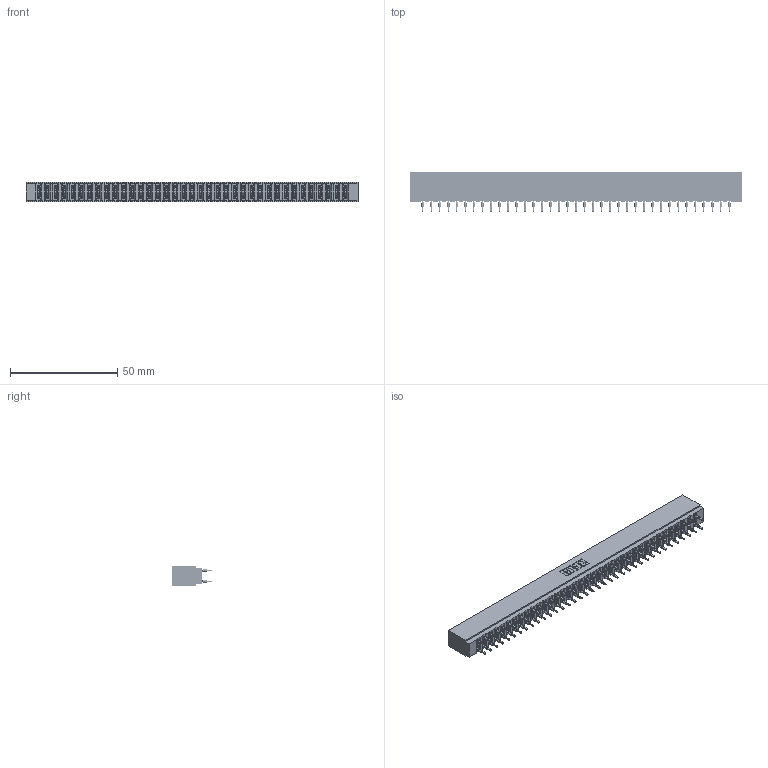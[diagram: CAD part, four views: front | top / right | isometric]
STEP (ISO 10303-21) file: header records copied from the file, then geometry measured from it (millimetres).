
FILE_DESCRIPTION (( 'STEP AP203' ), '1' );
FILE_NAME ('717-074-560-201.STEP', '2026-02-20T19:14:07', ( '' ), ( '' ), 'SwSTEP 2.0', 'SolidWorks 2023', '' );
FILE_SCHEMA (( 'CONFIG_CONTROL_DESIGN' ));
Length unit declared in the file: millimetre
Products named in the file (3): 717 Part_Insulator Option - 06; 745-292-001_560; 717-074-560-201
Assembly tree (75 placements, depth 2):
  717-074-560-201
    717 Part_Insulator Option - 06
    745-292-001_560  x74
Bounding box: 154.48 x 18.78 x 8.89 mm (x, y, z)
Volume: 13680 mm3; surface area: 22161.9 mm2
Topology: 75 solids, 75 shells, 7420 faces, 20305 edges, 12894 vertices
Faces by surface type: plane 3865, cylinder 1631, bspline 1480, torus 444
Entity records: 64448 total; most frequent: CARTESIAN_POINT 11693, ORIENTED_EDGE 11118, DIRECTION 9715, EDGE_CURVE 5559, VECTOR 5147, LINE 5147, VERTEX_POINT 3550, AXIS2_PLACEMENT_3D 2284
